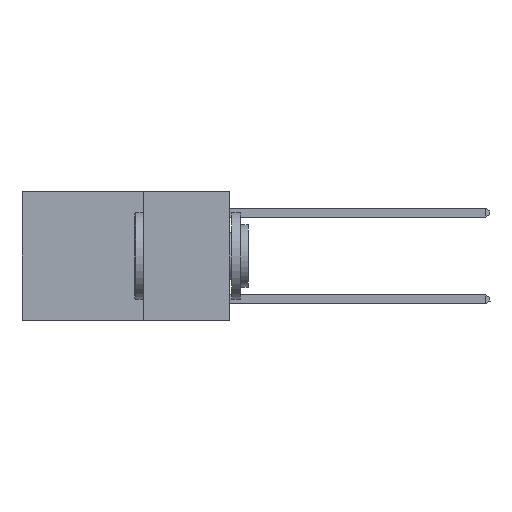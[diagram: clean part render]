
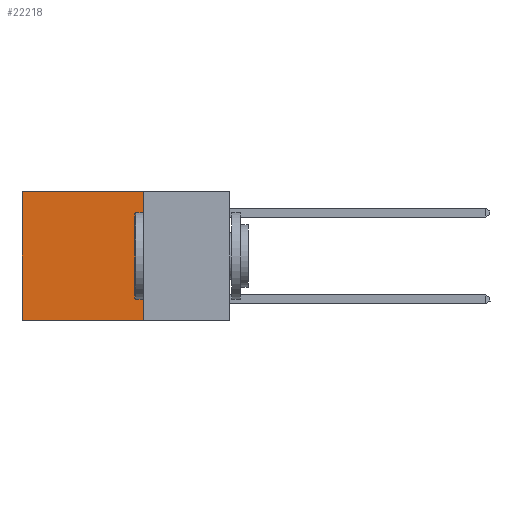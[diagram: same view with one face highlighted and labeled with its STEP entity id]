
A CAD part, left-side view. The second image highlights one B-rep face of the part: STEP entity #22218.
In plain terms, the highlighted planar face has unit normal (-1, 0, 0).
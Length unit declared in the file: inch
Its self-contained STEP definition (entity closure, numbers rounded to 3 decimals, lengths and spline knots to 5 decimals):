
#304 = CARTESIAN_POINT ( 'NONE',  ( 0.2625, 0.25, 0. ) ) ;
#1047 = VECTOR ( 'NONE', #14640, 39.37008 ) ;
#2433 = DIRECTION ( 'NONE',  ( 1., 0., 0. ) ) ;
#2761 = CARTESIAN_POINT ( 'NONE',  ( 0.2625, 0.25, 0. ) ) ;
#2818 = DIRECTION ( 'NONE',  ( 0., 0., -1. ) ) ;
#3621 = CARTESIAN_POINT ( 'NONE',  ( 0.2625, 0.25, 0. ) ) ;
#3623 = AXIS2_PLACEMENT_3D ( 'NONE', #304, #2433, #16271 ) ;
#4788 = CARTESIAN_POINT ( 'NONE',  ( 0.2625, 0.25, -0.37 ) ) ;
#4930 = CARTESIAN_POINT ( 'NONE',  ( 0.2625, 0.6, 0. ) ) ;
#5714 = CARTESIAN_POINT ( 'NONE',  ( 0.2625, 0.6, 0. ) ) ;
#6754 = VERTEX_POINT ( 'NONE', #24275 ) ;
#7058 = VERTEX_POINT ( 'NONE', #23165 ) ;
#7091 = EDGE_CURVE ( 'NONE', #21647, #6754, #11303, .T. ) ;
#7872 = FACE_OUTER_BOUND ( 'NONE', #14511, .T. ) ;
#8569 = VECTOR ( 'NONE', #16570, 39.37008 ) ;
#8727 = EDGE_CURVE ( 'NONE', #21581, #7058, #19833, .T. ) ;
#8873 = ORIENTED_EDGE ( 'NONE', *, *, #20551, .T. ) ;
#8985 = ORIENTED_EDGE ( 'NONE', *, *, #8727, .F. ) ;
#11303 = LINE ( 'NONE', #5714, #15950 ) ;
#11664 = LINE ( 'NONE', #2761, #1047 ) ;
#11751 = ORIENTED_EDGE ( 'NONE', *, *, #7091, .T. ) ;
#12662 = CARTESIAN_POINT ( 'NONE',  ( 0.2625, 0.25, 0. ) ) ;
#14320 = PLANE ( 'NONE',  #3623 ) ;
#14511 = EDGE_LOOP ( 'NONE', ( #11751, #18787, #8985, #8873 ) ) ;
#14640 = DIRECTION ( 'NONE',  ( 0., 1., 0. ) ) ;
#14702 = VECTOR ( 'NONE', #2818, 39.37008 ) ;
#14724 = EDGE_CURVE ( 'NONE', #7058, #6754, #20238, .T. ) ;
#15950 = VECTOR ( 'NONE', #19439, 39.37008 ) ;
#16271 = DIRECTION ( 'NONE',  ( 0., 0., -1. ) ) ;
#16570 = DIRECTION ( 'NONE',  ( 0., 1., 0. ) ) ;
#18787 = ORIENTED_EDGE ( 'NONE', *, *, #14724, .F. ) ;
#19439 = DIRECTION ( 'NONE',  ( 0., 0., -1. ) ) ;
#19833 = LINE ( 'NONE', #12662, #14702 ) ;
#20238 = LINE ( 'NONE', #4788, #8569 ) ;
#20551 = EDGE_CURVE ( 'NONE', #21581, #21647, #11664, .T. ) ;
#21581 = VERTEX_POINT ( 'NONE', #3621 ) ;
#21647 = VERTEX_POINT ( 'NONE', #4930 ) ;
#22218 = ADVANCED_FACE ( 'NONE', ( #7872 ), #14320, .F. ) ;
#23165 = CARTESIAN_POINT ( 'NONE',  ( 0.2625, 0.25, -0.37 ) ) ;
#24275 = CARTESIAN_POINT ( 'NONE',  ( 0.2625, 0.6, -0.37 ) ) ;
